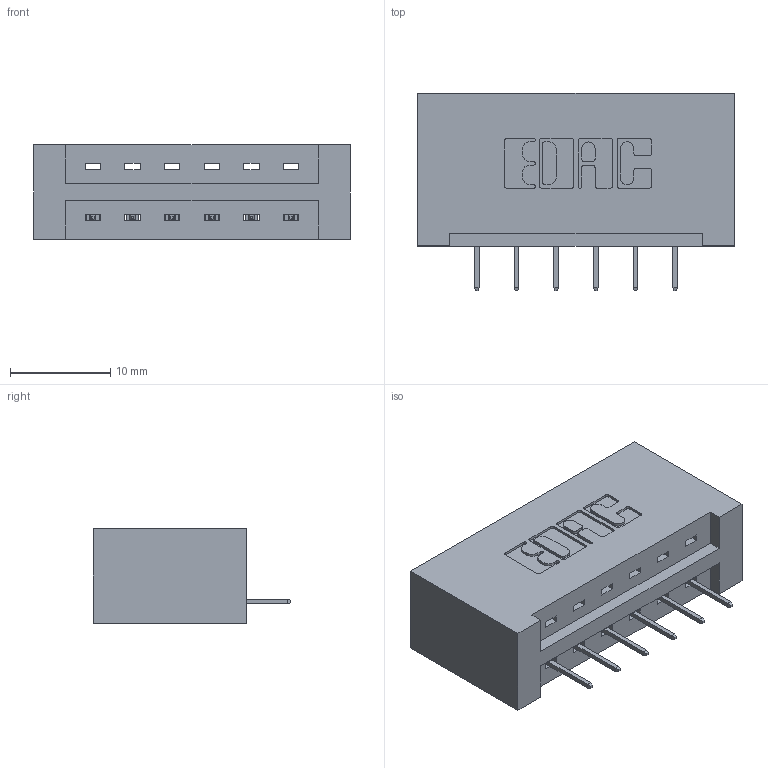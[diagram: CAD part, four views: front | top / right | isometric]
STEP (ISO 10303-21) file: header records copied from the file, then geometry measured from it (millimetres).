
FILE_DESCRIPTION (( 'STEP AP203' ), '1' );
FILE_NAME ('337-006-524-101.STEP', '2019-09-27T16:56:40', ( '' ), ( '' ), 'SwSTEP 2.0', 'SolidWorks 2016', '' );
FILE_SCHEMA (( 'CONFIG_CONTROL_DESIGN' ));
Length unit declared in the file: inch
Products named in the file (3): 337-006-524-101; 337 Part_No Mounting Lugs; 345-292-001_345-293-124
Assembly tree (7 placements, depth 2):
  337-006-524-101
    337 Part_No Mounting Lugs
    345-292-001_345-293-124  x6
Bounding box: 31.65 x 19.69 x 9.4 mm (x, y, z)
Volume: 3553.8 mm3; surface area: 3370.6 mm2
Topology: 7 solids, 7 shells, 502 faces, 1439 edges, 934 vertices
Faces by surface type: plane 378, cylinder 124
Entity records: 8913 total; most frequent: CARTESIAN_POINT 1556, ORIENTED_EDGE 1498, DIRECTION 1377, EDGE_CURVE 749, VECTOR 633, LINE 633, VERTEX_POINT 494, AXIS2_PLACEMENT_3D 372
